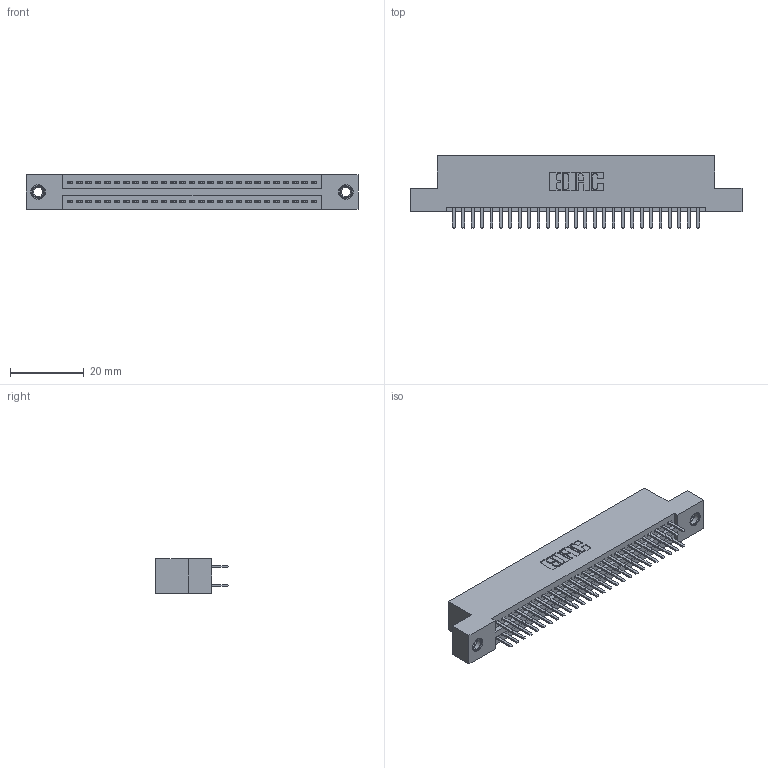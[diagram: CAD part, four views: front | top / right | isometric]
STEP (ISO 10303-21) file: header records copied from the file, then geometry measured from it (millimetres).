
FILE_DESCRIPTION (( 'STEP AP203' ), '1' );
FILE_NAME ('395-054-520-207.STEP', '2018-11-21T06:06:50', ( '' ), ( '' ), 'SwSTEP 2.0', 'SolidWorks 2016', '' );
FILE_SCHEMA (( 'CONFIG_CONTROL_DESIGN' ));
Length unit declared in the file: inch
Products named in the file (4): 345-250-001_345-250-005-103; 395-054-520-207; 345 Part_Flush Mounting Lugs - 0.156 Dia-TI; 345-292-001_345-293-120
Assembly tree (57 placements, depth 2):
  395-054-520-207
    345 Part_Flush Mounting Lugs - 0.156 Dia-TI
    345-292-001_345-293-120  x54
    345-250-001_345-250-005-103  x2
Bounding box: 89.79 x 19.68 x 9.4 mm (x, y, z)
Volume: 8545.7 mm3; surface area: 12318.9 mm2
Topology: 57 solids, 57 shells, 3102 faces, 8955 edges, 5818 vertices
Faces by surface type: plane 2002, cylinder 1084, cone 12, torus 4
Entity records: 24504 total; most frequent: CARTESIAN_POINT 4115, ORIENTED_EDGE 4030, DIRECTION 3661, EDGE_CURVE 2015, VECTOR 1751, LINE 1751, VERTEX_POINT 1336, AXIS2_PLACEMENT_3D 955
